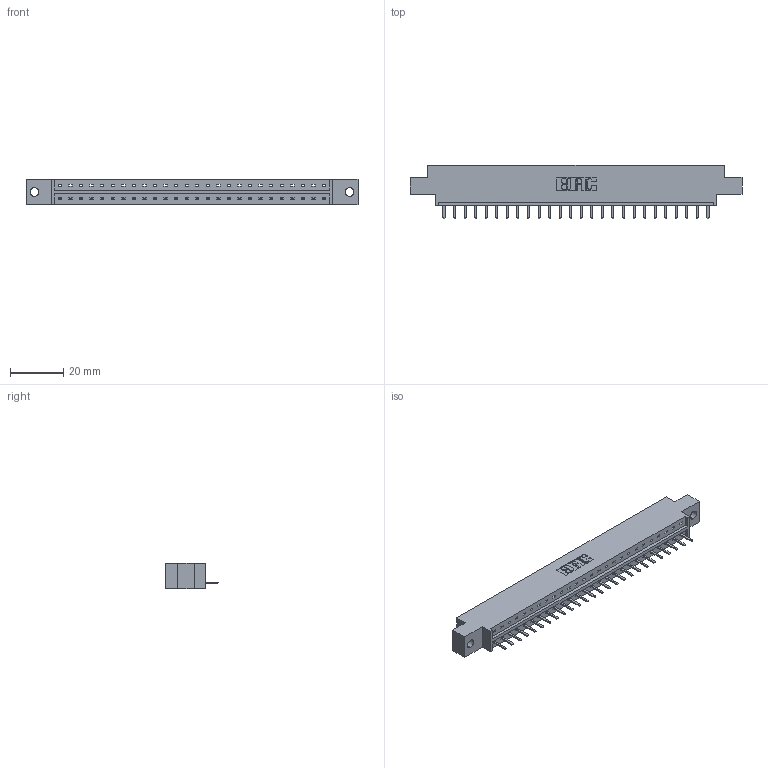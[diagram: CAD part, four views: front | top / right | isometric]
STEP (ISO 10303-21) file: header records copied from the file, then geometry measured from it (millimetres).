
FILE_DESCRIPTION (( 'STEP AP203' ), '1' );
FILE_NAME ('833-026-520-602.STEP', '2020-06-02T00:45:45', ( '' ), ( '' ), 'SwSTEP 2.0', 'SolidWorks 2020', '' );
FILE_SCHEMA (( 'CONFIG_CONTROL_DESIGN' ));
Length unit declared in the file: inch
Products named in the file (3): 833-026-520-602; 833 Part_Offset - .128 Dia; 345-292-001_345-293-120
Assembly tree (27 placements, depth 2):
  833-026-520-602
    833 Part_Offset - .128 Dia
    345-292-001_345-293-120  x26
Bounding box: 124.56 x 20.02 x 9.4 mm (x, y, z)
Volume: 12057.5 mm3; surface area: 12604.7 mm2
Topology: 27 solids, 27 shells, 1730 faces, 5107 edges, 3334 vertices
Faces by surface type: plane 1218, cylinder 512
Entity records: 18213 total; most frequent: CARTESIAN_POINT 3164, ORIENTED_EDGE 3114, DIRECTION 2689, EDGE_CURVE 1557, LINE 1425, VECTOR 1425, VERTEX_POINT 1034, AXIS2_PLACEMENT_3D 632
